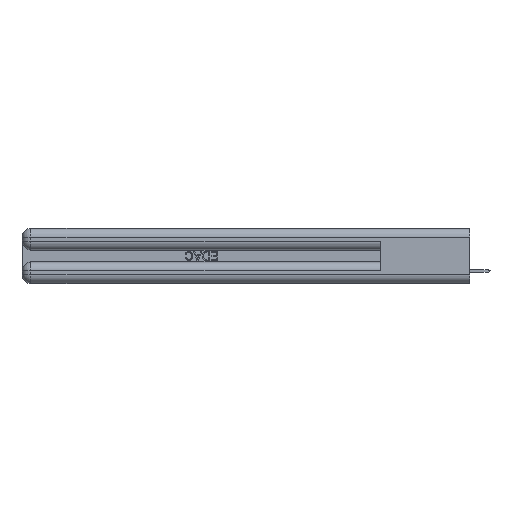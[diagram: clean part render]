
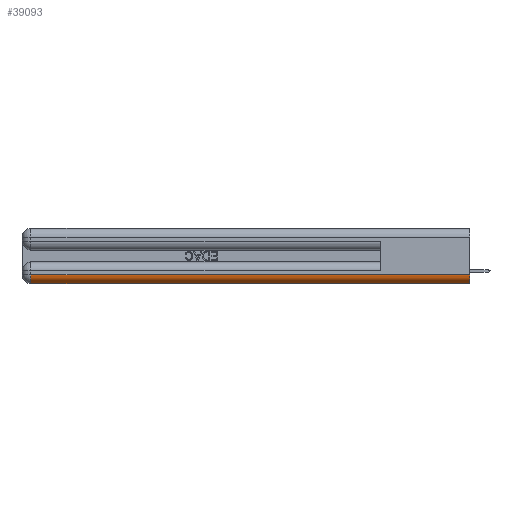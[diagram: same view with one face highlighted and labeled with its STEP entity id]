
A CAD part, left-side view. The second image highlights one B-rep face of the part: STEP entity #39093.
In plain terms, the highlighted cylindrical face has radius 1.524 mm (diameter 3.048 mm), a partial arc.
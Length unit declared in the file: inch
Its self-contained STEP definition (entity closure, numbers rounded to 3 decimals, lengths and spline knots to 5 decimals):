
#736 = EDGE_CURVE ( 'NONE', #11280, #8314, #15787, .T. ) ;
#2043 = CIRCLE ( 'NONE', #17603, 0.06 ) ;
#2061 = DIRECTION ( 'NONE',  ( 0., 1., 0. ) ) ;
#3215 = CARTESIAN_POINT ( 'NONE',  ( 0.06, 0., 0. ) ) ;
#4757 = LINE ( 'NONE', #35336, #30752 ) ;
#5399 = EDGE_CURVE ( 'NONE', #31988, #13485, #2043, .T. ) ;
#6637 = EDGE_CURVE ( 'NONE', #8314, #31988, #20297, .T. ) ;
#6886 = CARTESIAN_POINT ( 'NONE',  ( 0.06, 0., 0.06 ) ) ;
#7097 = CYLINDRICAL_SURFACE ( 'NONE', #9516, 0.06 ) ;
#8314 = VERTEX_POINT ( 'NONE', #3215 ) ;
#9516 = AXIS2_PLACEMENT_3D ( 'NONE', #6886, #28302, #10122 ) ;
#10059 = CARTESIAN_POINT ( 'NONE',  ( 0.06, 0., 0.06 ) ) ;
#10122 = DIRECTION ( 'NONE',  ( 0., 0., 1. ) ) ;
#11280 = VERTEX_POINT ( 'NONE', #26067 ) ;
#11884 = AXIS2_PLACEMENT_3D ( 'NONE', #10059, #25030, #27839 ) ;
#11972 = DIRECTION ( 'NONE',  ( 0., 0., 1. ) ) ;
#12054 = ORIENTED_EDGE ( 'NONE', *, *, #736, .F. ) ;
#12199 = FACE_OUTER_BOUND ( 'NONE', #12595, .T. ) ;
#12595 = EDGE_LOOP ( 'NONE', ( #12054, #25666, #29907, #27885 ) ) ;
#13485 = VERTEX_POINT ( 'NONE', #18947 ) ;
#15787 = CIRCLE ( 'NONE', #11884, 0.06 ) ;
#17603 = AXIS2_PLACEMENT_3D ( 'NONE', #30377, #36452, #11972 ) ;
#18947 = CARTESIAN_POINT ( 'NONE',  ( 0., 2.94, 0.06 ) ) ;
#20297 = LINE ( 'NONE', #38868, #20856 ) ;
#20856 = VECTOR ( 'NONE', #2061, 39.37008 ) ;
#21766 = EDGE_CURVE ( 'NONE', #13485, #11280, #4757, .T. ) ;
#25030 = DIRECTION ( 'NONE',  ( 0., -1., 0. ) ) ;
#25666 = ORIENTED_EDGE ( 'NONE', *, *, #21766, .F. ) ;
#26067 = CARTESIAN_POINT ( 'NONE',  ( 0., 0., 0.06 ) ) ;
#27839 = DIRECTION ( 'NONE',  ( 0., 0., 1. ) ) ;
#27885 = ORIENTED_EDGE ( 'NONE', *, *, #6637, .F. ) ;
#28302 = DIRECTION ( 'NONE',  ( 0., 1., 0. ) ) ;
#29907 = ORIENTED_EDGE ( 'NONE', *, *, #5399, .F. ) ;
#30377 = CARTESIAN_POINT ( 'NONE',  ( 0.06, 2.94, 0.06 ) ) ;
#30752 = VECTOR ( 'NONE', #36138, 39.37008 ) ;
#31988 = VERTEX_POINT ( 'NONE', #32000 ) ;
#32000 = CARTESIAN_POINT ( 'NONE',  ( 0.06, 2.94, 0. ) ) ;
#35336 = CARTESIAN_POINT ( 'NONE',  ( 0., 0., 0.06 ) ) ;
#36138 = DIRECTION ( 'NONE',  ( 0., -1., 0. ) ) ;
#36452 = DIRECTION ( 'NONE',  ( 0., 1., 0. ) ) ;
#38868 = CARTESIAN_POINT ( 'NONE',  ( 0.06, 3., 0. ) ) ;
#39093 = ADVANCED_FACE ( 'NONE', ( #12199 ), #7097, .T. ) ;
